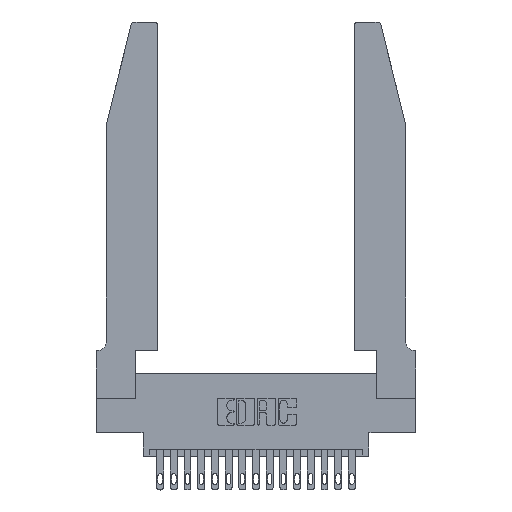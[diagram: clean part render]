
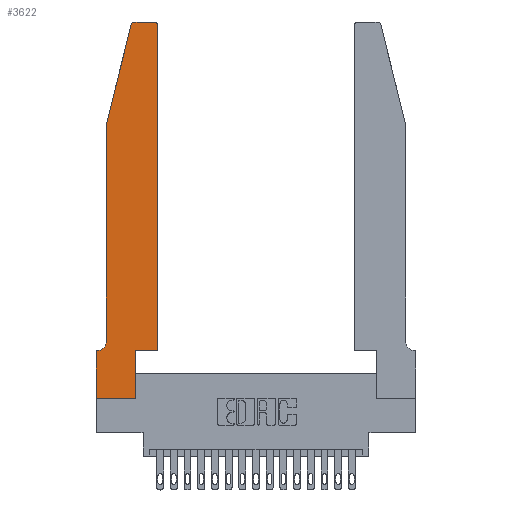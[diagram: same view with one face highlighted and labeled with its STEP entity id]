
A CAD part, top view. The second image highlights one B-rep face of the part: STEP entity #3622.
In plain terms, the highlighted planar face has unit normal (0, 0, 1).
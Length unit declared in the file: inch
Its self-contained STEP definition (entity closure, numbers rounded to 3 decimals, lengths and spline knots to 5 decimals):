
#304 = LINE ( 'NONE', #6796, #10559 ) ;
#348 = DIRECTION ( 'NONE',  ( 1., 0., 0. ) ) ;
#549 = VERTEX_POINT ( 'NONE', #9110 ) ;
#701 = DIRECTION ( 'NONE',  ( -1., 0., 0. ) ) ;
#916 = VERTEX_POINT ( 'NONE', #17365 ) ;
#932 = CARTESIAN_POINT ( 'NONE',  ( 0.0755, 0.35, 0.37 ) ) ;
#979 = AXIS2_PLACEMENT_3D ( 'NONE', #9927, #10056, #701 ) ;
#1262 = CARTESIAN_POINT ( 'NONE',  ( 0.0755, 2., 0.37 ) ) ;
#1329 = VECTOR ( 'NONE', #2670, 39.37008 ) ;
#1511 = AXIS2_PLACEMENT_3D ( 'NONE', #6699, #2124, #348 ) ;
#1964 = DIRECTION ( 'NONE',  ( 1., 0., 0. ) ) ;
#2041 = CIRCLE ( 'NONE', #1511, 0.03 ) ;
#2124 = DIRECTION ( 'NONE',  ( 0., 0., 1. ) ) ;
#2650 = CARTESIAN_POINT ( 'NONE',  ( 0.0755, 2., 0.37 ) ) ;
#2656 = CARTESIAN_POINT ( 'NONE',  ( 0.2865, 0.35, 0.37 ) ) ;
#2668 = VECTOR ( 'NONE', #10722, 39.37008 ) ;
#2670 = DIRECTION ( 'NONE',  ( 1., 0., 0. ) ) ;
#2711 = LINE ( 'NONE', #2650, #12435 ) ;
#2712 = VERTEX_POINT ( 'NONE', #2656 ) ;
#2725 = ORIENTED_EDGE ( 'NONE', *, *, #3200, .T. ) ;
#2901 = DIRECTION ( 'NONE',  ( 1., 0., 0. ) ) ;
#3200 = EDGE_CURVE ( 'NONE', #549, #916, #19206, .T. ) ;
#3462 = ORIENTED_EDGE ( 'NONE', *, *, #9857, .T. ) ;
#3622 = ADVANCED_FACE ( 'NONE', ( #9672 ), #14556, .T. ) ;
#3714 = CARTESIAN_POINT ( 'NONE',  ( 0., 0.35, 0.37 ) ) ;
#3841 = ORIENTED_EDGE ( 'NONE', *, *, #18701, .T. ) ;
#4137 = VERTEX_POINT ( 'NONE', #6572 ) ;
#4147 = DIRECTION ( 'NONE',  ( -1., 0., 0. ) ) ;
#4156 = CARTESIAN_POINT ( 'NONE',  ( 0., 0., 0.37 ) ) ;
#4532 = LINE ( 'NONE', #18591, #13771 ) ;
#5174 = CARTESIAN_POINT ( 'NONE',  ( 0.0755, 0.42, 0.37 ) ) ;
#5482 = LINE ( 'NONE', #4156, #1329 ) ;
#5521 = CARTESIAN_POINT ( 'NONE',  ( 0.4505, 0.35, 0.37 ) ) ;
#5831 = EDGE_CURVE ( 'NONE', #916, #18223, #2041, .T. ) ;
#6572 = CARTESIAN_POINT ( 'NONE',  ( 0., 0., 0.37 ) ) ;
#6658 = DIRECTION ( 'NONE',  ( 0., 0., 1. ) ) ;
#6699 = CARTESIAN_POINT ( 'NONE',  ( 0.284, 2.72, 0.37 ) ) ;
#6796 = CARTESIAN_POINT ( 'NONE',  ( 0.2865, 0.35, 0.37 ) ) ;
#6967 = VERTEX_POINT ( 'NONE', #14620 ) ;
#6981 = EDGE_CURVE ( 'NONE', #14167, #13707, #15184, .T. ) ;
#8071 = CIRCLE ( 'NONE', #15254, 0.03 ) ;
#8084 = DIRECTION ( 'NONE',  ( 0., 1., 0. ) ) ;
#8113 = VECTOR ( 'NONE', #11539, 39.37008 ) ;
#8356 = CARTESIAN_POINT ( 'NONE',  ( 0.0755, 2., 0.37 ) ) ;
#8359 = DIRECTION ( 'NONE',  ( 1., 0., 0. ) ) ;
#8479 = VERTEX_POINT ( 'NONE', #16291 ) ;
#8646 = ORIENTED_EDGE ( 'NONE', *, *, #9288, .T. ) ;
#8921 = DIRECTION ( 'NONE',  ( 0., -1., 0. ) ) ;
#9110 = CARTESIAN_POINT ( 'NONE',  ( 0.4205, 2.75, 0.37 ) ) ;
#9124 = ORIENTED_EDGE ( 'NONE', *, *, #17599, .T. ) ;
#9241 = CARTESIAN_POINT ( 'NONE',  ( 0., 0., 0.37 ) ) ;
#9288 = EDGE_CURVE ( 'NONE', #2712, #8479, #4532, .T. ) ;
#9623 = DIRECTION ( 'NONE',  ( 0., 0., 1. ) ) ;
#9672 = FACE_OUTER_BOUND ( 'NONE', #17934, .T. ) ;
#9857 = EDGE_CURVE ( 'NONE', #4137, #11989, #5482, .T. ) ;
#9927 = CARTESIAN_POINT ( 'NONE',  ( 0.0055, 0.42, 0.37 ) ) ;
#10056 = DIRECTION ( 'NONE',  ( 0., 0., -1. ) ) ;
#10288 = LINE ( 'NONE', #932, #17879 ) ;
#10559 = VECTOR ( 'NONE', #8084, 39.37008 ) ;
#10574 = VERTEX_POINT ( 'NONE', #1262 ) ;
#10722 = DIRECTION ( 'NONE',  ( 0., -1., 0. ) ) ;
#11313 = CARTESIAN_POINT ( 'NONE',  ( 0.0055, 0.35, 0.37 ) ) ;
#11355 = CARTESIAN_POINT ( 'NONE',  ( 0.4205, 2.72, 0.37 ) ) ;
#11369 = ORIENTED_EDGE ( 'NONE', *, *, #5831, .T. ) ;
#11539 = DIRECTION ( 'NONE',  ( -0.239, -0.971, 0. ) ) ;
#11989 = VERTEX_POINT ( 'NONE', #19666 ) ;
#12431 = ORIENTED_EDGE ( 'NONE', *, *, #17430, .T. ) ;
#12435 = VECTOR ( 'NONE', #8921, 39.37008 ) ;
#12922 = VECTOR ( 'NONE', #17956, 39.37008 ) ;
#13707 = VERTEX_POINT ( 'NONE', #11313 ) ;
#13728 = VERTEX_POINT ( 'NONE', #18977 ) ;
#13771 = VECTOR ( 'NONE', #2901, 39.37008 ) ;
#13885 = AXIS2_PLACEMENT_3D ( 'NONE', #3714, #6658, #8359 ) ;
#13951 = LINE ( 'NONE', #8356, #8113 ) ;
#14167 = VERTEX_POINT ( 'NONE', #5174 ) ;
#14556 = PLANE ( 'NONE',  #13885 ) ;
#14620 = CARTESIAN_POINT ( 'NONE',  ( 0.4505, 2.72, 0.37 ) ) ;
#14728 = ORIENTED_EDGE ( 'NONE', *, *, #6981, .T. ) ;
#15184 = CIRCLE ( 'NONE', #979, 0.07 ) ;
#15254 = AXIS2_PLACEMENT_3D ( 'NONE', #11355, #9623, #1964 ) ;
#15354 = LINE ( 'NONE', #9241, #2668 ) ;
#15783 = ORIENTED_EDGE ( 'NONE', *, *, #17046, .T. ) ;
#16291 = CARTESIAN_POINT ( 'NONE',  ( 0.4505, 0.35, 0.37 ) ) ;
#16629 = LINE ( 'NONE', #5521, #12922 ) ;
#16665 = ORIENTED_EDGE ( 'NONE', *, *, #20098, .T. ) ;
#16835 = EDGE_CURVE ( 'NONE', #13707, #13728, #10288, .T. ) ;
#17046 = EDGE_CURVE ( 'NONE', #6967, #549, #8071, .T. ) ;
#17191 = ORIENTED_EDGE ( 'NONE', *, *, #20090, .T. ) ;
#17365 = CARTESIAN_POINT ( 'NONE',  ( 0.284, 2.75, 0.37 ) ) ;
#17377 = CARTESIAN_POINT ( 'NONE',  ( 0.25487, 2.72718, 0.37 ) ) ;
#17430 = EDGE_CURVE ( 'NONE', #10574, #14167, #2711, .T. ) ;
#17599 = EDGE_CURVE ( 'NONE', #8479, #6967, #16629, .T. ) ;
#17747 = VECTOR ( 'NONE', #4147, 39.37008 ) ;
#17879 = VECTOR ( 'NONE', #19584, 39.37008 ) ;
#17934 = EDGE_LOOP ( 'NONE', ( #2725, #11369, #16665, #12431, #14728, #20134, #3841, #3462, #17191, #8646, #9124, #15783 ) ) ;
#17956 = DIRECTION ( 'NONE',  ( 0., 1., 0. ) ) ;
#18223 = VERTEX_POINT ( 'NONE', #17377 ) ;
#18366 = CARTESIAN_POINT ( 'NONE',  ( 0.2605, 2.75, 0.37 ) ) ;
#18591 = CARTESIAN_POINT ( 'NONE',  ( 0.4505, 0.35, 0.37 ) ) ;
#18701 = EDGE_CURVE ( 'NONE', #13728, #4137, #15354, .T. ) ;
#18977 = CARTESIAN_POINT ( 'NONE',  ( 0., 0.35, 0.37 ) ) ;
#19206 = LINE ( 'NONE', #18366, #17747 ) ;
#19584 = DIRECTION ( 'NONE',  ( -1., 0., 0. ) ) ;
#19666 = CARTESIAN_POINT ( 'NONE',  ( 0.2865, 0., 0.37 ) ) ;
#20090 = EDGE_CURVE ( 'NONE', #11989, #2712, #304, .T. ) ;
#20098 = EDGE_CURVE ( 'NONE', #18223, #10574, #13951, .T. ) ;
#20134 = ORIENTED_EDGE ( 'NONE', *, *, #16835, .T. ) ;
